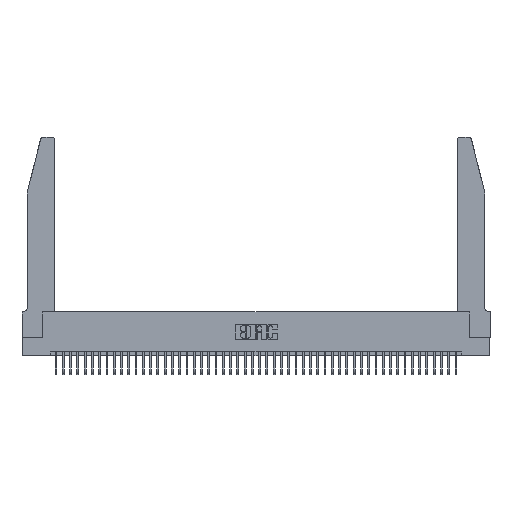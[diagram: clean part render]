
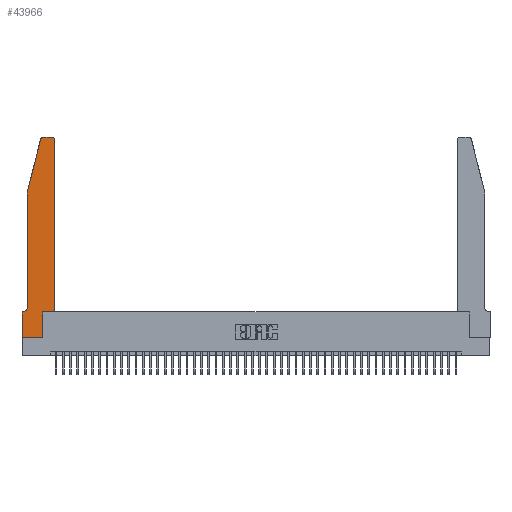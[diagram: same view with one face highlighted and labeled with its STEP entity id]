
A CAD part, top view. The second image highlights one B-rep face of the part: STEP entity #43966.
In plain terms, the highlighted planar face has unit normal (0, 0, 1).
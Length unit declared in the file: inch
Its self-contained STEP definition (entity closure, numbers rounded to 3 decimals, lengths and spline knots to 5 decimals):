
#2586 = VERTEX_POINT ( 'NONE', #44266 ) ;
#2676 = EDGE_CURVE ( 'NONE', #24220, #24501, #26901, .T. ) ;
#3376 = AXIS2_PLACEMENT_3D ( 'NONE', #46089, #12530, #16284 ) ;
#3617 = VERTEX_POINT ( 'NONE', #4500 ) ;
#4500 = CARTESIAN_POINT ( 'NONE',  ( 0.284, 2.75, 0.37 ) ) ;
#4778 = ORIENTED_EDGE ( 'NONE', *, *, #15367, .T. ) ;
#5506 = CIRCLE ( 'NONE', #3376, 0.03 ) ;
#5656 = DIRECTION ( 'NONE',  ( -1., 0., 0. ) ) ;
#5822 = VECTOR ( 'NONE', #32226, 39.37008 ) ;
#7247 = VECTOR ( 'NONE', #33208, 39.37008 ) ;
#8465 = VERTEX_POINT ( 'NONE', #31616 ) ;
#9378 = LINE ( 'NONE', #24364, #5822 ) ;
#9615 = DIRECTION ( 'NONE',  ( 0., 1., 0. ) ) ;
#10355 = DIRECTION ( 'NONE',  ( 1., 0., 0. ) ) ;
#10579 = EDGE_CURVE ( 'NONE', #13878, #8465, #24625, .T. ) ;
#12166 = LINE ( 'NONE', #46781, #15084 ) ;
#12530 = DIRECTION ( 'NONE',  ( 0., 0., 1. ) ) ;
#12651 = VERTEX_POINT ( 'NONE', #21150 ) ;
#13291 = LINE ( 'NONE', #29020, #25611 ) ;
#13351 = ORIENTED_EDGE ( 'NONE', *, *, #42187, .T. ) ;
#13557 = DIRECTION ( 'NONE',  ( 1., 0., 0. ) ) ;
#13878 = VERTEX_POINT ( 'NONE', #20963 ) ;
#14879 = EDGE_CURVE ( 'NONE', #22034, #2586, #25888, .T. ) ;
#15084 = VECTOR ( 'NONE', #9615, 39.37008 ) ;
#15288 = ORIENTED_EDGE ( 'NONE', *, *, #29210, .T. ) ;
#15367 = EDGE_CURVE ( 'NONE', #2586, #42026, #30450, .T. ) ;
#15876 = VECTOR ( 'NONE', #43211, 39.37008 ) ;
#15939 = EDGE_CURVE ( 'NONE', #12651, #3617, #22459, .T. ) ;
#16284 = DIRECTION ( 'NONE',  ( 1., 0., 0. ) ) ;
#16638 = DIRECTION ( 'NONE',  ( 0., 0., -1. ) ) ;
#16651 = CARTESIAN_POINT ( 'NONE',  ( 0.0755, 2., 0.37 ) ) ;
#17001 = VECTOR ( 'NONE', #36932, 39.37008 ) ;
#17222 = LINE ( 'NONE', #29461, #7247 ) ;
#17639 = CARTESIAN_POINT ( 'NONE',  ( 0.4505, 2.72, 0.37 ) ) ;
#18657 = DIRECTION ( 'NONE',  ( -0.239, -0.971, 0. ) ) ;
#18769 = ORIENTED_EDGE ( 'NONE', *, *, #48133, .T. ) ;
#18816 = EDGE_CURVE ( 'NONE', #24501, #13878, #9378, .T. ) ;
#19741 = EDGE_CURVE ( 'NONE', #44073, #12651, #32133, .T. ) ;
#20050 = DIRECTION ( 'NONE',  ( 1., 0., 0. ) ) ;
#20240 = ORIENTED_EDGE ( 'NONE', *, *, #19741, .T. ) ;
#20777 = PLANE ( 'NONE',  #46414 ) ;
#20963 = CARTESIAN_POINT ( 'NONE',  ( 0.0755, 0.42, 0.37 ) ) ;
#21150 = CARTESIAN_POINT ( 'NONE',  ( 0.4205, 2.75, 0.37 ) ) ;
#21335 = CARTESIAN_POINT ( 'NONE',  ( 0.2605, 2.75, 0.37 ) ) ;
#21982 = DIRECTION ( 'NONE',  ( -1., 0., 0. ) ) ;
#22034 = VERTEX_POINT ( 'NONE', #45952 ) ;
#22388 = FACE_OUTER_BOUND ( 'NONE', #40106, .T. ) ;
#22459 = LINE ( 'NONE', #21335, #28911 ) ;
#22471 = ORIENTED_EDGE ( 'NONE', *, *, #15939, .T. ) ;
#23147 = VERTEX_POINT ( 'NONE', #35048 ) ;
#24220 = VERTEX_POINT ( 'NONE', #24939 ) ;
#24364 = CARTESIAN_POINT ( 'NONE',  ( 0.0755, 2., 0.37 ) ) ;
#24501 = VERTEX_POINT ( 'NONE', #45633 ) ;
#24625 = CIRCLE ( 'NONE', #34827, 0.07 ) ;
#24928 = ORIENTED_EDGE ( 'NONE', *, *, #14879, .T. ) ;
#24939 = CARTESIAN_POINT ( 'NONE',  ( 0.25487, 2.72718, 0.37 ) ) ;
#25611 = VECTOR ( 'NONE', #10355, 39.37008 ) ;
#25888 = LINE ( 'NONE', #43055, #15876 ) ;
#26901 = LINE ( 'NONE', #16651, #31012 ) ;
#27112 = CARTESIAN_POINT ( 'NONE',  ( 0.4205, 2.72, 0.37 ) ) ;
#28307 = DIRECTION ( 'NONE',  ( 0., 0., 1. ) ) ;
#28911 = VECTOR ( 'NONE', #21982, 39.37008 ) ;
#29020 = CARTESIAN_POINT ( 'NONE',  ( 0., 0., 0.37 ) ) ;
#29210 = EDGE_CURVE ( 'NONE', #46798, #23147, #17222, .T. ) ;
#29461 = CARTESIAN_POINT ( 'NONE',  ( 0., 0., 0.37 ) ) ;
#30210 = ORIENTED_EDGE ( 'NONE', *, *, #2676, .T. ) ;
#30400 = ORIENTED_EDGE ( 'NONE', *, *, #18816, .T. ) ;
#30450 = LINE ( 'NONE', #37599, #42181 ) ;
#31012 = VECTOR ( 'NONE', #18657, 39.37008 ) ;
#31616 = CARTESIAN_POINT ( 'NONE',  ( 0.0055, 0.35, 0.37 ) ) ;
#31800 = EDGE_CURVE ( 'NONE', #8465, #46798, #38710, .T. ) ;
#32133 = CIRCLE ( 'NONE', #32900, 0.03 ) ;
#32226 = DIRECTION ( 'NONE',  ( 0., -1., 0. ) ) ;
#32900 = AXIS2_PLACEMENT_3D ( 'NONE', #27112, #38914, #20050 ) ;
#33208 = DIRECTION ( 'NONE',  ( 0., -1., 0. ) ) ;
#33891 = EDGE_CURVE ( 'NONE', #23147, #22034, #13291, .T. ) ;
#33970 = CARTESIAN_POINT ( 'NONE',  ( 0.4505, 0.35, 0.37 ) ) ;
#34827 = AXIS2_PLACEMENT_3D ( 'NONE', #39062, #16638, #5656 ) ;
#35048 = CARTESIAN_POINT ( 'NONE',  ( 0., 0., 0.37 ) ) ;
#36779 = CARTESIAN_POINT ( 'NONE',  ( 0.0755, 0.35, 0.37 ) ) ;
#36932 = DIRECTION ( 'NONE',  ( -1., 0., 0. ) ) ;
#37599 = CARTESIAN_POINT ( 'NONE',  ( 0.4505, 0.35, 0.37 ) ) ;
#38710 = LINE ( 'NONE', #36779, #17001 ) ;
#38914 = DIRECTION ( 'NONE',  ( 0., 0., 1. ) ) ;
#39062 = CARTESIAN_POINT ( 'NONE',  ( 0.0055, 0.42, 0.37 ) ) ;
#40106 = EDGE_LOOP ( 'NONE', ( #22471, #13351, #30210, #30400, #48327, #48071, #15288, #41343, #24928, #4778, #18769, #20240 ) ) ;
#41343 = ORIENTED_EDGE ( 'NONE', *, *, #33891, .T. ) ;
#42026 = VERTEX_POINT ( 'NONE', #33970 ) ;
#42181 = VECTOR ( 'NONE', #45114, 39.37008 ) ;
#42187 = EDGE_CURVE ( 'NONE', #3617, #24220, #5506, .T. ) ;
#42864 = CARTESIAN_POINT ( 'NONE',  ( 0., 0.35, 0.37 ) ) ;
#43055 = CARTESIAN_POINT ( 'NONE',  ( 0.2865, 0.35, 0.37 ) ) ;
#43211 = DIRECTION ( 'NONE',  ( 0., 1., 0. ) ) ;
#43966 = ADVANCED_FACE ( 'NONE', ( #22388 ), #20777, .T. ) ;
#44073 = VERTEX_POINT ( 'NONE', #17639 ) ;
#44266 = CARTESIAN_POINT ( 'NONE',  ( 0.2865, 0.35, 0.37 ) ) ;
#45114 = DIRECTION ( 'NONE',  ( 1., 0., 0. ) ) ;
#45633 = CARTESIAN_POINT ( 'NONE',  ( 0.0755, 2., 0.37 ) ) ;
#45952 = CARTESIAN_POINT ( 'NONE',  ( 0.2865, 0., 0.37 ) ) ;
#46089 = CARTESIAN_POINT ( 'NONE',  ( 0.284, 2.72, 0.37 ) ) ;
#46363 = CARTESIAN_POINT ( 'NONE',  ( 0., 0.35, 0.37 ) ) ;
#46414 = AXIS2_PLACEMENT_3D ( 'NONE', #42864, #28307, #13557 ) ;
#46781 = CARTESIAN_POINT ( 'NONE',  ( 0.4505, 0.35, 0.37 ) ) ;
#46798 = VERTEX_POINT ( 'NONE', #46363 ) ;
#48071 = ORIENTED_EDGE ( 'NONE', *, *, #31800, .T. ) ;
#48133 = EDGE_CURVE ( 'NONE', #42026, #44073, #12166, .T. ) ;
#48327 = ORIENTED_EDGE ( 'NONE', *, *, #10579, .T. ) ;
